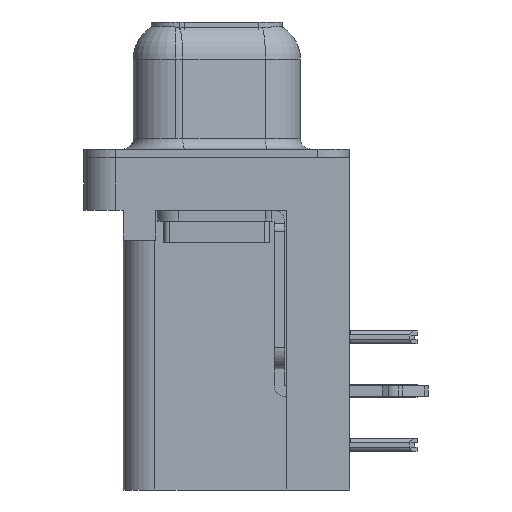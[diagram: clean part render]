
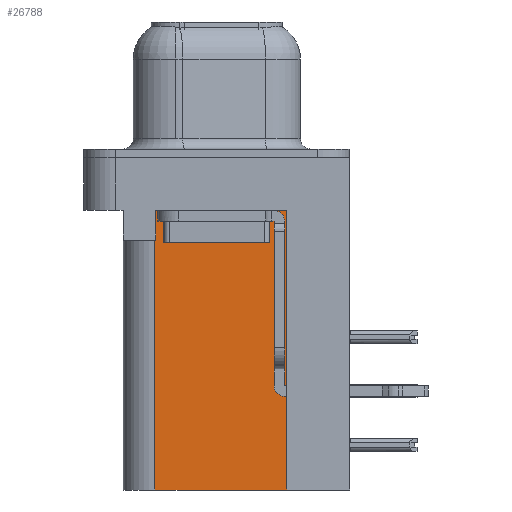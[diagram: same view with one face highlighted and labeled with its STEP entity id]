
A CAD part, left-side view. The second image highlights one B-rep face of the part: STEP entity #26788.
In plain terms, the highlighted planar face has unit normal (-1, 0, 0).
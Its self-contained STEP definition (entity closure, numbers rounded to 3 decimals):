
#564 = VECTOR ( 'NONE', #34035, 1000. ) ;
#1163 = VERTEX_POINT ( 'NONE', #19469 ) ;
#1498 = LINE ( 'NONE', #36709, #564 ) ;
#2172 = CARTESIAN_POINT ( 'NONE',  ( 3.765, 2.925, -3.9 ) ) ;
#2481 = ORIENTED_EDGE ( 'NONE', *, *, #15423, .T. ) ;
#2851 = VECTOR ( 'NONE', #33819, 1000. ) ;
#3298 = DIRECTION ( 'NONE',  ( 0., 0., -1. ) ) ;
#4469 = ORIENTED_EDGE ( 'NONE', *, *, #20117, .T. ) ;
#4588 = CARTESIAN_POINT ( 'NONE',  ( 3.765, 2.895, -2.5 ) ) ;
#4589 = DIRECTION ( 'NONE',  ( 0., 0., -1. ) ) ;
#7028 = EDGE_LOOP ( 'NONE', ( #2481, #13276, #16636, #34743, #15933, #4469 ) ) ;
#8764 = CARTESIAN_POINT ( 'NONE',  ( 3.765, 0., -3.9 ) ) ;
#9824 = LINE ( 'NONE', #8764, #33708 ) ;
#10919 = EDGE_CURVE ( 'NONE', #18205, #20202, #28319, .T. ) ;
#11292 = EDGE_CURVE ( 'NONE', #20202, #15043, #9824, .T. ) ;
#11611 = CARTESIAN_POINT ( 'NONE',  ( 3.765, -3.295, -2.5 ) ) ;
#11750 = DIRECTION ( 'NONE',  ( 0., 1., 0. ) ) ;
#13276 = ORIENTED_EDGE ( 'NONE', *, *, #10919, .T. ) ;
#14781 = VECTOR ( 'NONE', #21395, 1000. ) ;
#15043 = VERTEX_POINT ( 'NONE', #2172 ) ;
#15196 = FACE_OUTER_BOUND ( 'NONE', #7028, .T. ) ;
#15423 = EDGE_CURVE ( 'NONE', #32358, #18205, #32907, .T. ) ;
#15933 = ORIENTED_EDGE ( 'NONE', *, *, #23851, .F. ) ;
#16636 = ORIENTED_EDGE ( 'NONE', *, *, #11292, .T. ) ;
#17314 = AXIS2_PLACEMENT_3D ( 'NONE', #36378, #22277, #4589 ) ;
#18205 = VERTEX_POINT ( 'NONE', #4588 ) ;
#19375 = PLANE ( 'NONE',  #17314 ) ;
#19469 = CARTESIAN_POINT ( 'NONE',  ( 3.765, 2.925, -15.7 ) ) ;
#20117 = EDGE_CURVE ( 'NONE', #21115, #32358, #37407, .T. ) ;
#20202 = VERTEX_POINT ( 'NONE', #30266 ) ;
#21115 = VERTEX_POINT ( 'NONE', #36325 ) ;
#21244 = CARTESIAN_POINT ( 'NONE',  ( 3.765, -3.295, -15.7 ) ) ;
#21395 = DIRECTION ( 'NONE',  ( 0., 0., 1. ) ) ;
#21723 = VECTOR ( 'NONE', #3298, 1000. ) ;
#22277 = DIRECTION ( 'NONE',  ( 1., 0., 0. ) ) ;
#23851 = EDGE_CURVE ( 'NONE', #21115, #1163, #25219, .T. ) ;
#23895 = CARTESIAN_POINT ( 'NONE',  ( 3.765, 2.895, -3.9 ) ) ;
#25219 = LINE ( 'NONE', #29988, #32730 ) ;
#26788 = ADVANCED_FACE ( 'NONE', ( #15196 ), #19375, .F. ) ;
#28319 = LINE ( 'NONE', #23895, #21723 ) ;
#29988 = CARTESIAN_POINT ( 'NONE',  ( 3.765, -3.295, -15.7 ) ) ;
#30266 = CARTESIAN_POINT ( 'NONE',  ( 3.765, 2.895, -3.9 ) ) ;
#30838 = EDGE_CURVE ( 'NONE', #1163, #15043, #1498, .T. ) ;
#32358 = VERTEX_POINT ( 'NONE', #11611 ) ;
#32730 = VECTOR ( 'NONE', #35777, 1000. ) ;
#32907 = LINE ( 'NONE', #36615, #2851 ) ;
#33708 = VECTOR ( 'NONE', #11750, 1000. ) ;
#33819 = DIRECTION ( 'NONE',  ( 0., 1., 0. ) ) ;
#34035 = DIRECTION ( 'NONE',  ( 0., 0., 1. ) ) ;
#34743 = ORIENTED_EDGE ( 'NONE', *, *, #30838, .F. ) ;
#35777 = DIRECTION ( 'NONE',  ( 0., 1., 0. ) ) ;
#36325 = CARTESIAN_POINT ( 'NONE',  ( 3.765, -3.295, -15.7 ) ) ;
#36378 = CARTESIAN_POINT ( 'NONE',  ( 3.765, -3.295, -15.7 ) ) ;
#36615 = CARTESIAN_POINT ( 'NONE',  ( 3.765, -3.295, -2.5 ) ) ;
#36709 = CARTESIAN_POINT ( 'NONE',  ( 3.765, 2.925, -15.7 ) ) ;
#37407 = LINE ( 'NONE', #21244, #14781 ) ;
